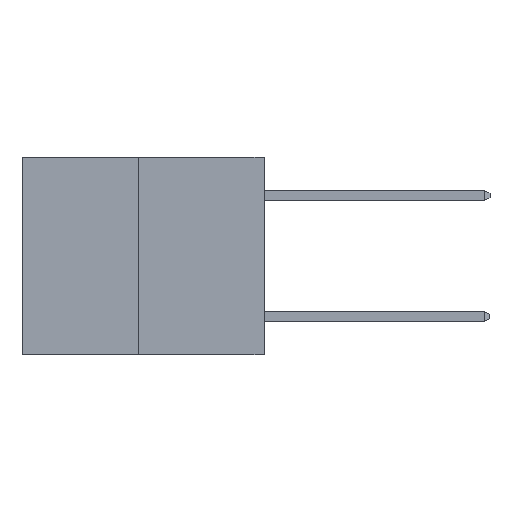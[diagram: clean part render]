
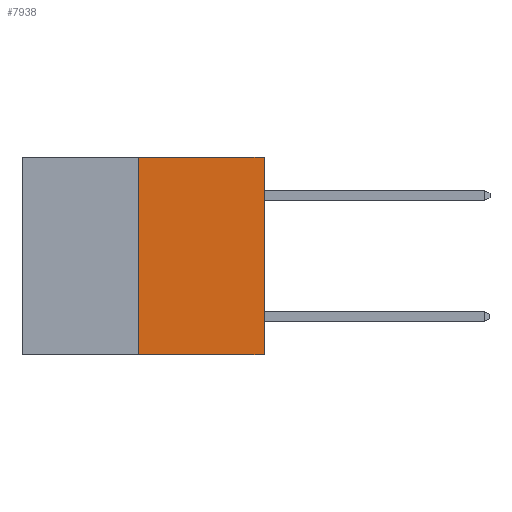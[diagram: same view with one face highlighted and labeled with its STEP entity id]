
A CAD part, left-side view. The second image highlights one B-rep face of the part: STEP entity #7938.
In plain terms, the highlighted planar face has unit normal (-1, 0, 0).
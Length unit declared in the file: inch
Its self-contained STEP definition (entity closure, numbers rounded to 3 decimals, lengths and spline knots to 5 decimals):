
#422 = PLANE ( 'NONE',  #3073 ) ;
#605 = CARTESIAN_POINT ( 'NONE',  ( 0., 0.6, 0. ) ) ;
#1140 = VERTEX_POINT ( 'NONE', #10226 ) ;
#2625 = VECTOR ( 'NONE', #5167, 39.37008 ) ;
#2694 = DIRECTION ( 'NONE',  ( 0., -1., 0. ) ) ;
#3073 = AXIS2_PLACEMENT_3D ( 'NONE', #9582, #7330, #5050 ) ;
#3143 = VECTOR ( 'NONE', #2694, 39.37008 ) ;
#3166 = EDGE_LOOP ( 'NONE', ( #12154, #13397, #6470, #10198 ) ) ;
#3476 = EDGE_CURVE ( 'NONE', #1140, #14309, #13438, .T. ) ;
#3796 = EDGE_CURVE ( 'NONE', #13934, #14309, #4067, .T. ) ;
#4067 = LINE ( 'NONE', #7357, #2625 ) ;
#4228 = LINE ( 'NONE', #14369, #3143 ) ;
#4545 = FACE_OUTER_BOUND ( 'NONE', #3166, .T. ) ;
#5050 = DIRECTION ( 'NONE',  ( 0., 0., -1. ) ) ;
#5167 = DIRECTION ( 'NONE',  ( 0., 0., 1. ) ) ;
#6470 = ORIENTED_EDGE ( 'NONE', *, *, #3796, .T. ) ;
#6501 = EDGE_CURVE ( 'NONE', #14884, #13934, #4228, .T. ) ;
#6521 = CARTESIAN_POINT ( 'NONE',  ( 0., 0., -0.49 ) ) ;
#6788 = LINE ( 'NONE', #10857, #11119 ) ;
#7330 = DIRECTION ( 'NONE',  ( 1., 0., 0. ) ) ;
#7357 = CARTESIAN_POINT ( 'NONE',  ( 0., 0., 0. ) ) ;
#7938 = ADVANCED_FACE ( 'NONE', ( #4545 ), #422, .F. ) ;
#8172 = VECTOR ( 'NONE', #13342, 39.37008 ) ;
#9582 = CARTESIAN_POINT ( 'NONE',  ( 0., 0.6, 0. ) ) ;
#9806 = DIRECTION ( 'NONE',  ( 0., 0., 1. ) ) ;
#9983 = EDGE_CURVE ( 'NONE', #14884, #1140, #6788, .T. ) ;
#10198 = ORIENTED_EDGE ( 'NONE', *, *, #3476, .F. ) ;
#10226 = CARTESIAN_POINT ( 'NONE',  ( 0., 0.312, 0. ) ) ;
#10857 = CARTESIAN_POINT ( 'NONE',  ( 0., 0.312, -0.49 ) ) ;
#11119 = VECTOR ( 'NONE', #9806, 39.37008 ) ;
#11560 = CARTESIAN_POINT ( 'NONE',  ( 0., 0., 0. ) ) ;
#12154 = ORIENTED_EDGE ( 'NONE', *, *, #9983, .F. ) ;
#12331 = CARTESIAN_POINT ( 'NONE',  ( 0., 0.312, -0.49 ) ) ;
#13342 = DIRECTION ( 'NONE',  ( 0., -1., 0. ) ) ;
#13397 = ORIENTED_EDGE ( 'NONE', *, *, #6501, .T. ) ;
#13438 = LINE ( 'NONE', #605, #8172 ) ;
#13934 = VERTEX_POINT ( 'NONE', #6521 ) ;
#14309 = VERTEX_POINT ( 'NONE', #11560 ) ;
#14369 = CARTESIAN_POINT ( 'NONE',  ( 0., 0.6, -0.49 ) ) ;
#14884 = VERTEX_POINT ( 'NONE', #12331 ) ;
